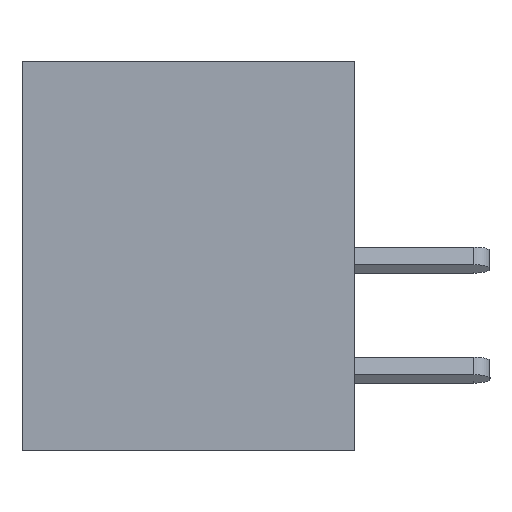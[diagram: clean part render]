
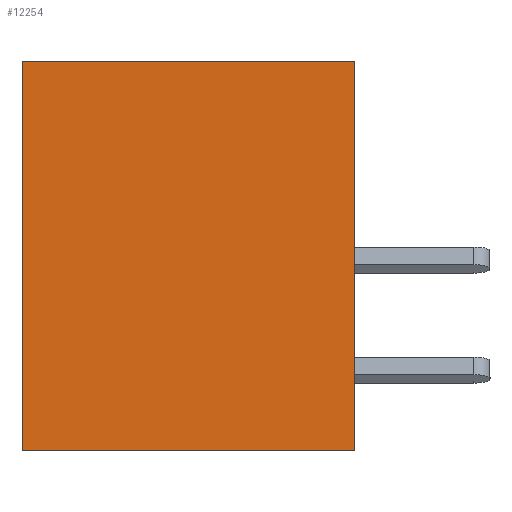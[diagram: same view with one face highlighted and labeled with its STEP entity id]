
A CAD part, left-side view. The second image highlights one B-rep face of the part: STEP entity #12254.
In plain terms, the highlighted planar face has unit normal (-1, 0, 0).
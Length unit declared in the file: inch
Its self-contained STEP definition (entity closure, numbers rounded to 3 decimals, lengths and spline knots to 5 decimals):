
#546 = ORIENTED_EDGE ( 'NONE', *, *, #4935, .T. ) ;
#1174 = EDGE_CURVE ( 'NONE', #8259, #3183, #16006, .T. ) ;
#1415 = CARTESIAN_POINT ( 'NONE',  ( 0., 0., 0. ) ) ;
#1945 = CARTESIAN_POINT ( 'NONE',  ( 0., 0., -0.531 ) ) ;
#2053 = VECTOR ( 'NONE', #11824, 39.37008 ) ;
#2177 = CARTESIAN_POINT ( 'NONE',  ( 0., 0., 0. ) ) ;
#3183 = VERTEX_POINT ( 'NONE', #2177 ) ;
#3548 = CARTESIAN_POINT ( 'NONE',  ( 0., 0.453, -0.531 ) ) ;
#4150 = DIRECTION ( 'NONE',  ( 1., 0., 0. ) ) ;
#4853 = EDGE_LOOP ( 'NONE', ( #6186, #13253, #10338, #546 ) ) ;
#4935 = EDGE_CURVE ( 'NONE', #16954, #11769, #11583, .T. ) ;
#5770 = DIRECTION ( 'NONE',  ( 0., 0., 1. ) ) ;
#6186 = ORIENTED_EDGE ( 'NONE', *, *, #14593, .T. ) ;
#6514 = CARTESIAN_POINT ( 'NONE',  ( 0., 0.453, 0. ) ) ;
#6720 = CARTESIAN_POINT ( 'NONE',  ( 0., 0.453, 0. ) ) ;
#6994 = EDGE_CURVE ( 'NONE', #16954, #8259, #7893, .T. ) ;
#7665 = FACE_OUTER_BOUND ( 'NONE', #4853, .T. ) ;
#7730 = CARTESIAN_POINT ( 'NONE',  ( 0., 0.453, -0.531 ) ) ;
#7888 = CARTESIAN_POINT ( 'NONE',  ( 0., 0.453, 0. ) ) ;
#7893 = LINE ( 'NONE', #12310, #9708 ) ;
#7945 = DIRECTION ( 'NONE',  ( 0., 0., -1. ) ) ;
#8259 = VERTEX_POINT ( 'NONE', #6720 ) ;
#9708 = VECTOR ( 'NONE', #5770, 39.37008 ) ;
#10338 = ORIENTED_EDGE ( 'NONE', *, *, #6994, .F. ) ;
#11583 = LINE ( 'NONE', #7730, #15864 ) ;
#11769 = VERTEX_POINT ( 'NONE', #1945 ) ;
#11824 = DIRECTION ( 'NONE',  ( 0., -1., 0. ) ) ;
#11891 = PLANE ( 'NONE',  #15186 ) ;
#12254 = ADVANCED_FACE ( 'NONE', ( #7665 ), #11891, .F. ) ;
#12310 = CARTESIAN_POINT ( 'NONE',  ( 0., 0.453, 0. ) ) ;
#13253 = ORIENTED_EDGE ( 'NONE', *, *, #1174, .F. ) ;
#13338 = DIRECTION ( 'NONE',  ( 0., 0., 1. ) ) ;
#14483 = LINE ( 'NONE', #1415, #16758 ) ;
#14593 = EDGE_CURVE ( 'NONE', #11769, #3183, #14483, .T. ) ;
#15186 = AXIS2_PLACEMENT_3D ( 'NONE', #7888, #4150, #7945 ) ;
#15695 = DIRECTION ( 'NONE',  ( 0., -1., 0. ) ) ;
#15864 = VECTOR ( 'NONE', #15695, 39.37008 ) ;
#16006 = LINE ( 'NONE', #6514, #2053 ) ;
#16758 = VECTOR ( 'NONE', #13338, 39.37008 ) ;
#16954 = VERTEX_POINT ( 'NONE', #3548 ) ;
